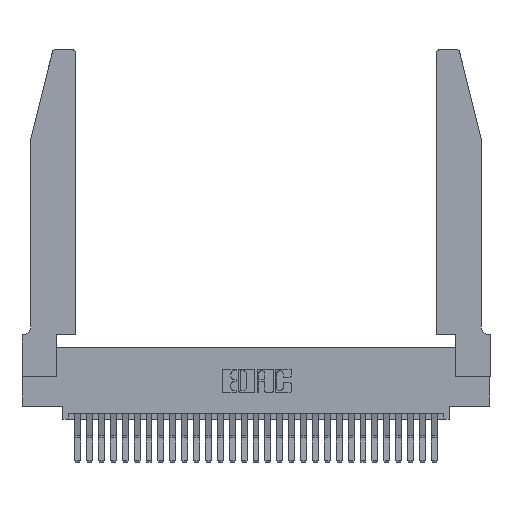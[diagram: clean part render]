
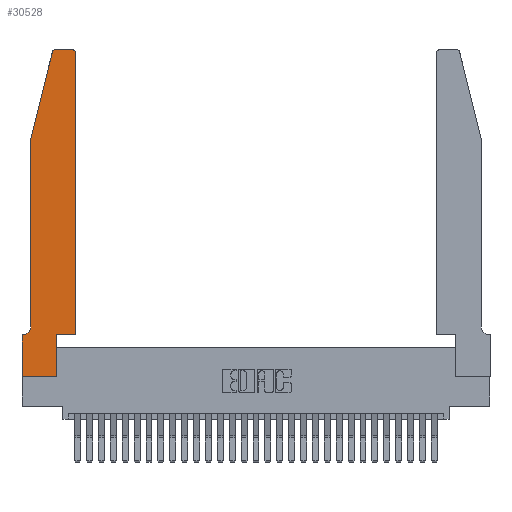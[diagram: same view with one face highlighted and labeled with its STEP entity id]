
A CAD part, top view. The second image highlights one B-rep face of the part: STEP entity #30528.
In plain terms, the highlighted planar face has unit normal (0, 0, 1).
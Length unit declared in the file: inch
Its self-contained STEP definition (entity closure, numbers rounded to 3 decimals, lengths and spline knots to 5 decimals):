
#164 = VERTEX_POINT ( 'NONE', #14277 ) ;
#251 = DIRECTION ( 'NONE',  ( -1., 0., 0. ) ) ;
#801 = VERTEX_POINT ( 'NONE', #6153 ) ;
#820 = EDGE_CURVE ( 'NONE', #22054, #7957, #4196, .T. ) ;
#1864 = LINE ( 'NONE', #13555, #7604 ) ;
#1916 = EDGE_CURVE ( 'NONE', #11563, #22054, #14641, .T. ) ;
#3399 = CARTESIAN_POINT ( 'NONE',  ( 0.284, 2.72, 0.37 ) ) ;
#3661 = CIRCLE ( 'NONE', #14441, 0.03 ) ;
#4080 = DIRECTION ( 'NONE',  ( -0.239, -0.971, 0. ) ) ;
#4196 = LINE ( 'NONE', #21341, #16181 ) ;
#4745 = DIRECTION ( 'NONE',  ( 1., 0., 0. ) ) ;
#4773 = CARTESIAN_POINT ( 'NONE',  ( 0.0055, 0.35, 0.37 ) ) ;
#5832 = VERTEX_POINT ( 'NONE', #6960 ) ;
#5862 = DIRECTION ( 'NONE',  ( 1., 0., 0. ) ) ;
#6153 = CARTESIAN_POINT ( 'NONE',  ( 0., 0.35, 0.37 ) ) ;
#6539 = VECTOR ( 'NONE', #15587, 39.37008 ) ;
#6688 = CARTESIAN_POINT ( 'NONE',  ( 0.2865, 0.35, 0.37 ) ) ;
#6960 = CARTESIAN_POINT ( 'NONE',  ( 0.25487, 2.72718, 0.37 ) ) ;
#7604 = VECTOR ( 'NONE', #15921, 39.37008 ) ;
#7673 = LINE ( 'NONE', #13643, #24969 ) ;
#7763 = DIRECTION ( 'NONE',  ( 0., 0., 1. ) ) ;
#7848 = ORIENTED_EDGE ( 'NONE', *, *, #9811, .T. ) ;
#7957 = VERTEX_POINT ( 'NONE', #22445 ) ;
#8101 = ORIENTED_EDGE ( 'NONE', *, *, #12749, .T. ) ;
#8380 = VERTEX_POINT ( 'NONE', #26315 ) ;
#9811 = EDGE_CURVE ( 'NONE', #13519, #11563, #13701, .T. ) ;
#9816 = ORIENTED_EDGE ( 'NONE', *, *, #29112, .T. ) ;
#9944 = EDGE_CURVE ( 'NONE', #28196, #801, #22470, .T. ) ;
#10092 = FACE_OUTER_BOUND ( 'NONE', #16931, .T. ) ;
#10600 = DIRECTION ( 'NONE',  ( 1., 0., 0. ) ) ;
#10851 = CARTESIAN_POINT ( 'NONE',  ( 0., 0., 0.37 ) ) ;
#11213 = CARTESIAN_POINT ( 'NONE',  ( 0.2605, 2.75, 0.37 ) ) ;
#11348 = VECTOR ( 'NONE', #23777, 39.37008 ) ;
#11563 = VERTEX_POINT ( 'NONE', #6688 ) ;
#11935 = VERTEX_POINT ( 'NONE', #29433 ) ;
#12298 = CIRCLE ( 'NONE', #26321, 0.03 ) ;
#12749 = EDGE_CURVE ( 'NONE', #18252, #18480, #19628, .T. ) ;
#12922 = LINE ( 'NONE', #10851, #6539 ) ;
#13519 = VERTEX_POINT ( 'NONE', #26150 ) ;
#13555 = CARTESIAN_POINT ( 'NONE',  ( 0., 0., 0.37 ) ) ;
#13643 = CARTESIAN_POINT ( 'NONE',  ( 0.0755, 2., 0.37 ) ) ;
#13701 = LINE ( 'NONE', #22035, #25394 ) ;
#14277 = CARTESIAN_POINT ( 'NONE',  ( 0.0755, 2., 0.37 ) ) ;
#14441 = AXIS2_PLACEMENT_3D ( 'NONE', #3399, #20053, #5862 ) ;
#14641 = LINE ( 'NONE', #20047, #20861 ) ;
#14734 = DIRECTION ( 'NONE',  ( 0., 0., -1. ) ) ;
#15237 = ORIENTED_EDGE ( 'NONE', *, *, #16957, .T. ) ;
#15532 = EDGE_CURVE ( 'NONE', #801, #8380, #12922, .T. ) ;
#15587 = DIRECTION ( 'NONE',  ( 0., -1., 0. ) ) ;
#15921 = DIRECTION ( 'NONE',  ( 1., 0., 0. ) ) ;
#16181 = VECTOR ( 'NONE', #26916, 39.37008 ) ;
#16282 = VECTOR ( 'NONE', #20202, 39.37008 ) ;
#16553 = EDGE_CURVE ( 'NONE', #164, #11935, #23791, .T. ) ;
#16653 = PLANE ( 'NONE',  #23500 ) ;
#16838 = CARTESIAN_POINT ( 'NONE',  ( 0.4205, 2.75, 0.37 ) ) ;
#16931 = EDGE_LOOP ( 'NONE', ( #8101, #19368, #9816, #27085, #15237, #27595, #21758, #21730, #7848, #17248, #19692, #19095 ) ) ;
#16957 = EDGE_CURVE ( 'NONE', #11935, #28196, #19077, .T. ) ;
#17248 = ORIENTED_EDGE ( 'NONE', *, *, #1916, .T. ) ;
#17880 = CARTESIAN_POINT ( 'NONE',  ( 0.0755, 0.35, 0.37 ) ) ;
#17962 = EDGE_CURVE ( 'NONE', #8380, #13519, #1864, .T. ) ;
#18252 = VERTEX_POINT ( 'NONE', #16838 ) ;
#18480 = VERTEX_POINT ( 'NONE', #29407 ) ;
#18917 = VECTOR ( 'NONE', #22881, 39.37008 ) ;
#19015 = DIRECTION ( 'NONE',  ( 0., 0., 1. ) ) ;
#19077 = CIRCLE ( 'NONE', #24873, 0.07 ) ;
#19095 = ORIENTED_EDGE ( 'NONE', *, *, #20706, .T. ) ;
#19368 = ORIENTED_EDGE ( 'NONE', *, *, #25720, .T. ) ;
#19628 = LINE ( 'NONE', #11213, #18917 ) ;
#19692 = ORIENTED_EDGE ( 'NONE', *, *, #820, .T. ) ;
#20047 = CARTESIAN_POINT ( 'NONE',  ( 0.4505, 0.35, 0.37 ) ) ;
#20053 = DIRECTION ( 'NONE',  ( 0., 0., 1. ) ) ;
#20202 = DIRECTION ( 'NONE',  ( -1., 0., 0. ) ) ;
#20706 = EDGE_CURVE ( 'NONE', #7957, #18252, #12298, .T. ) ;
#20861 = VECTOR ( 'NONE', #10600, 39.37008 ) ;
#21341 = CARTESIAN_POINT ( 'NONE',  ( 0.4505, 0.35, 0.37 ) ) ;
#21730 = ORIENTED_EDGE ( 'NONE', *, *, #17962, .T. ) ;
#21758 = ORIENTED_EDGE ( 'NONE', *, *, #15532, .T. ) ;
#21879 = CARTESIAN_POINT ( 'NONE',  ( 0.4205, 2.72, 0.37 ) ) ;
#22035 = CARTESIAN_POINT ( 'NONE',  ( 0.2865, 0.35, 0.37 ) ) ;
#22054 = VERTEX_POINT ( 'NONE', #22305 ) ;
#22305 = CARTESIAN_POINT ( 'NONE',  ( 0.4505, 0.35, 0.37 ) ) ;
#22445 = CARTESIAN_POINT ( 'NONE',  ( 0.4505, 2.72, 0.37 ) ) ;
#22470 = LINE ( 'NONE', #17880, #16282 ) ;
#22881 = DIRECTION ( 'NONE',  ( -1., 0., 0. ) ) ;
#23500 = AXIS2_PLACEMENT_3D ( 'NONE', #30648, #19015, #4745 ) ;
#23777 = DIRECTION ( 'NONE',  ( 0., -1., 0. ) ) ;
#23791 = LINE ( 'NONE', #28552, #11348 ) ;
#24205 = DIRECTION ( 'NONE',  ( 1., 0., 0. ) ) ;
#24363 = DIRECTION ( 'NONE',  ( 0., 1., 0. ) ) ;
#24873 = AXIS2_PLACEMENT_3D ( 'NONE', #28775, #14734, #251 ) ;
#24969 = VECTOR ( 'NONE', #4080, 39.37008 ) ;
#25394 = VECTOR ( 'NONE', #24363, 39.37008 ) ;
#25720 = EDGE_CURVE ( 'NONE', #18480, #5832, #3661, .T. ) ;
#26150 = CARTESIAN_POINT ( 'NONE',  ( 0.2865, 0., 0.37 ) ) ;
#26315 = CARTESIAN_POINT ( 'NONE',  ( 0., 0., 0.37 ) ) ;
#26321 = AXIS2_PLACEMENT_3D ( 'NONE', #21879, #7763, #24205 ) ;
#26916 = DIRECTION ( 'NONE',  ( 0., 1., 0. ) ) ;
#27085 = ORIENTED_EDGE ( 'NONE', *, *, #16553, .T. ) ;
#27595 = ORIENTED_EDGE ( 'NONE', *, *, #9944, .T. ) ;
#28196 = VERTEX_POINT ( 'NONE', #4773 ) ;
#28552 = CARTESIAN_POINT ( 'NONE',  ( 0.0755, 2., 0.37 ) ) ;
#28775 = CARTESIAN_POINT ( 'NONE',  ( 0.0055, 0.42, 0.37 ) ) ;
#29112 = EDGE_CURVE ( 'NONE', #5832, #164, #7673, .T. ) ;
#29407 = CARTESIAN_POINT ( 'NONE',  ( 0.284, 2.75, 0.37 ) ) ;
#29433 = CARTESIAN_POINT ( 'NONE',  ( 0.0755, 0.42, 0.37 ) ) ;
#30528 = ADVANCED_FACE ( 'NONE', ( #10092 ), #16653, .T. ) ;
#30648 = CARTESIAN_POINT ( 'NONE',  ( 0., 0.35, 0.37 ) ) ;
